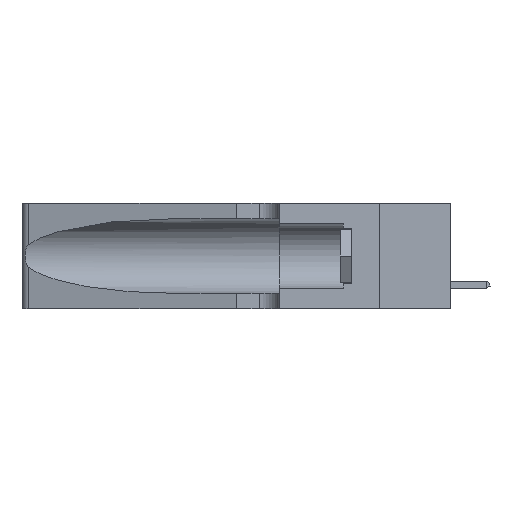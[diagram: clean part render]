
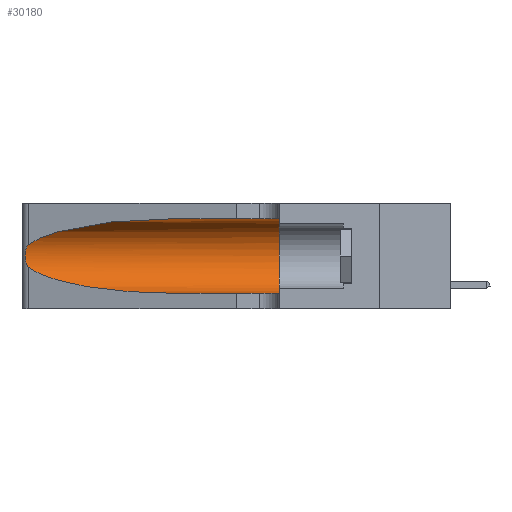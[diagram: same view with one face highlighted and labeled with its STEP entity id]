
A CAD part, left-side view. The second image highlights one B-rep face of the part: STEP entity #30180.
In plain terms, the highlighted cylindrical face has radius 3.308 mm (diameter 6.617 mm), a partial arc.
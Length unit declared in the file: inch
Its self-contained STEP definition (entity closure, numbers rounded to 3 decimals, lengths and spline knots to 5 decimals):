
#134 = B_SPLINE_CURVE_WITH_KNOTS ( 'NONE', 3,
 ( #16437, #19095, #17136, #6761, #21585, #5961, #12168, #7629, #2912, #3262, #11592, #28487, #28705, #33679 ),
 .UNSPECIFIED., .F., .F.,
 ( 4, 2, 2, 2, 2, 2, 4 ),
 ( 0., 0.00027, 0.00053, 0.00107, 0.0016, 0.00187, 0.00214 ),
 .UNSPECIFIED. ) ;
#597 = CARTESIAN_POINT ( 'NONE',  ( 0.1305, 1.61858, 0.31525 ) ) ;
#1100 = VERTEX_POINT ( 'NONE', #8229 ) ;
#2012 = CARTESIAN_POINT ( 'NONE',  ( 0.1305, 0.35, 0.31525 ) ) ;
#2912 = CARTESIAN_POINT ( 'NONE',  ( 0.26017, 1.23833, 0.17102 ) ) ;
#2935 = EDGE_CURVE ( 'NONE', #1100, #7317, #134, .T. ) ;
#3262 = CARTESIAN_POINT ( 'NONE',  ( 0.25856, 1.23593, 0.16098 ) ) ;
#4013 = CARTESIAN_POINT ( 'NONE',  ( 0.25487, 1.22718, 0.14631 ) ) ;
#4350 = CARTESIAN_POINT ( 'NONE',  ( 0.1305, 0.72297, 0.05475 ) ) ;
#4757 = DIRECTION ( 'NONE',  ( 0., -1., 0. ) ) ;
#5671 = CARTESIAN_POINT ( 'NONE',  ( 0.1305, 0.72297, 0.31525 ) ) ;
#5961 = CARTESIAN_POINT ( 'NONE',  ( 0.26018, 1.23835, 0.19895 ) ) ;
#6582 = DIRECTION ( 'NONE',  ( 0., -1., 0. ) ) ;
#6604 = VECTOR ( 'NONE', #4757, 39.37008 ) ;
#6624 = CARTESIAN_POINT ( 'NONE',  ( 0.25487, 1.22718, 0.14631 ) ) ;
#6761 = CARTESIAN_POINT ( 'NONE',  ( 0.25787, 1.23484, 0.2124 ) ) ;
#6822 = VERTEX_POINT ( 'NONE', #17571 ) ;
#7317 = VERTEX_POINT ( 'NONE', #6624 ) ;
#7629 = CARTESIAN_POINT ( 'NONE',  ( 0.26075, 1.23896, 0.178 ) ) ;
#8229 = CARTESIAN_POINT ( 'NONE',  ( 0.25487, 1.22718, 0.22369 ) ) ;
#8812 = DIRECTION ( 'NONE',  ( 0., 0., 1. ) ) ;
#9876 = VERTEX_POINT ( 'NONE', #11232 ) ;
#10195 = CARTESIAN_POINT ( 'NONE',  ( 0.1305, 1.61858, 0.05475 ) ) ;
#10581 = EDGE_CURVE ( 'NONE', #16125, #29626, #22452, .T. ) ;
#11182 = DIRECTION ( 'NONE',  ( 0., -1., 0. ) ) ;
#11232 = CARTESIAN_POINT ( 'NONE',  ( 0.1305, 0.72297, 0.31525 ) ) ;
#11592 = CARTESIAN_POINT ( 'NONE',  ( 0.25789, 1.23486, 0.15765 ) ) ;
#12168 = CARTESIAN_POINT ( 'NONE',  ( 0.26075, 1.23896, 0.19203 ) ) ;
#14250 = CARTESIAN_POINT ( 'NONE',  ( 0.1305, 0.35, 0.185 ) ) ;
#14316 = DIRECTION ( 'NONE',  ( 0., 0., -1. ) ) ;
#14850 = ORIENTED_EDGE ( 'NONE', *, *, #27083, .T. ) ;
#15145 = AXIS2_PLACEMENT_3D ( 'NONE', #14250, #22167, #8812 ) ;
#15326 = EDGE_LOOP ( 'NONE', ( #14850, #17636, #19175, #29369, #26528, #22853 ) ) ;
#15612 = LINE ( 'NONE', #597, #28709 ) ;
#16125 = VERTEX_POINT ( 'NONE', #2012 ) ;
#16437 = CARTESIAN_POINT ( 'NONE',  ( 0.25487, 1.22718, 0.22369 ) ) ;
#17011 = FACE_OUTER_BOUND ( 'NONE', #15326, .T. ) ;
#17136 = CARTESIAN_POINT ( 'NONE',  ( 0.25639, 1.23184, 0.21858 ) ) ;
#17571 = CARTESIAN_POINT ( 'NONE',  ( 0.1305, 0.72297, 0.05475 ) ) ;
#17636 = ORIENTED_EDGE ( 'NONE', *, *, #2935, .T. ) ;
#17659 = CARTESIAN_POINT ( 'NONE',  ( 0.25487, 1.22718, 0.22369 ) ) ;
#18031 = LINE ( 'NONE', #10195, #6604 ) ;
#18128 = EDGE_CURVE ( 'NONE', #7317, #6822, #26054, .T. ) ;
#19095 = CARTESIAN_POINT ( 'NONE',  ( 0.25555, 1.22994, 0.2215 ) ) ;
#19175 = ORIENTED_EDGE ( 'NONE', *, *, #18128, .T. ) ;
#19641 = CARTESIAN_POINT ( 'NONE',  ( 0.2373, 1.15595, 0.08982 ) ) ;
#19876 = CARTESIAN_POINT ( 'NONE',  ( 0.1305, 0.35, 0.05475 ) ) ;
#21361 = EDGE_CURVE ( 'NONE', #6822, #29626, #18031, .T. ) ;
#21585 = CARTESIAN_POINT ( 'NONE',  ( 0.25854, 1.2359, 0.20912 ) ) ;
#22167 = DIRECTION ( 'NONE',  ( 0., 1., 0. ) ) ;
#22271 = CARTESIAN_POINT ( 'NONE',  ( 0.18966, 0.96281, 0.05475 ) ) ;
#22452 = CIRCLE ( 'NONE', #15145, 0.13025 ) ;
#22568 = CARTESIAN_POINT ( 'NONE',  ( 0.2373, 1.15595, 0.28018 ) ) ;
#22853 = ORIENTED_EDGE ( 'NONE', *, *, #32184, .F. ) ;
#26054 =( BOUNDED_CURVE ( )  B_SPLINE_CURVE ( 3, ( #4013, #19641, #22271, #4350 ),
 .UNSPECIFIED., .F., .F. ) 
 B_SPLINE_CURVE_WITH_KNOTS ( ( 4, 4 ),
 ( 3.44316, 4.71239 ),
 .UNSPECIFIED. ) 
 CURVE ( )  GEOMETRIC_REPRESENTATION_ITEM ( )  RATIONAL_B_SPLINE_CURVE ( ( 1., 0.87, 0.87, 1. ) ) 
 REPRESENTATION_ITEM ( '' )  );
#26528 = ORIENTED_EDGE ( 'NONE', *, *, #10581, .F. ) ;
#27083 = EDGE_CURVE ( 'NONE', #9876, #1100, #27110, .T. ) ;
#27110 =( BOUNDED_CURVE ( )  B_SPLINE_CURVE ( 3, ( #5671, #29192, #22568, #17659 ),
 .UNSPECIFIED., .F., .T. ) 
 B_SPLINE_CURVE_WITH_KNOTS ( ( 4, 4 ),
 ( 1.5708, 2.84003 ),
 .UNSPECIFIED. ) 
 CURVE ( )  GEOMETRIC_REPRESENTATION_ITEM ( )  RATIONAL_B_SPLINE_CURVE ( ( 1., 0.87, 0.87, 1. ) ) 
 REPRESENTATION_ITEM ( '' )  );
#28487 = CARTESIAN_POINT ( 'NONE',  ( 0.25639, 1.23186, 0.15144 ) ) ;
#28705 = CARTESIAN_POINT ( 'NONE',  ( 0.25555, 1.22993, 0.14849 ) ) ;
#28709 = VECTOR ( 'NONE', #11182, 39.37008 ) ;
#29083 = AXIS2_PLACEMENT_3D ( 'NONE', #29982, #6582, #14316 ) ;
#29192 = CARTESIAN_POINT ( 'NONE',  ( 0.18966, 0.96281, 0.31525 ) ) ;
#29369 = ORIENTED_EDGE ( 'NONE', *, *, #21361, .T. ) ;
#29626 = VERTEX_POINT ( 'NONE', #19876 ) ;
#29982 = CARTESIAN_POINT ( 'NONE',  ( 0.1305, 1.61858, 0.185 ) ) ;
#30180 = ADVANCED_FACE ( 'NONE', ( #17011 ), #33673, .F. ) ;
#32184 = EDGE_CURVE ( 'NONE', #9876, #16125, #15612, .T. ) ;
#33673 = CYLINDRICAL_SURFACE ( 'NONE', #29083, 0.13025 ) ;
#33679 = CARTESIAN_POINT ( 'NONE',  ( 0.25487, 1.22718, 0.14631 ) ) ;
